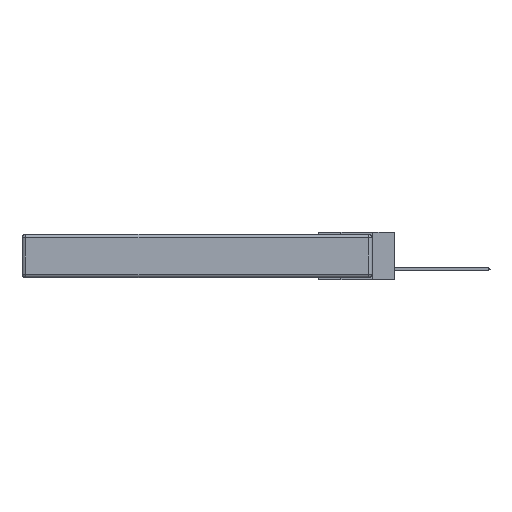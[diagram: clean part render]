
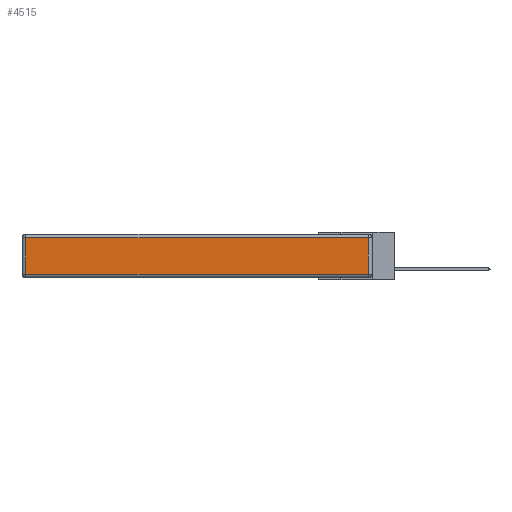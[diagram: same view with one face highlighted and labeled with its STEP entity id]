
A CAD part, left-side view. The second image highlights one B-rep face of the part: STEP entity #4515.
In plain terms, the highlighted planar face has unit normal (-1, 0, 0).
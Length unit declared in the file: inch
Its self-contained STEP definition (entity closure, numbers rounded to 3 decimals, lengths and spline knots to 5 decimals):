
#292 = ORIENTED_EDGE ( 'NONE', *, *, #18853, .T. ) ;
#667 = AXIS2_PLACEMENT_3D ( 'NONE', #30467, #11760, #16222 ) ;
#1671 = VERTEX_POINT ( 'NONE', #16600 ) ;
#2238 = DIRECTION ( 'NONE',  ( 0., -1., 0. ) ) ;
#3206 = VECTOR ( 'NONE', #18641, 39.37008 ) ;
#3739 = VERTEX_POINT ( 'NONE', #28798 ) ;
#4317 = VECTOR ( 'NONE', #6408, 39.37008 ) ;
#4515 = ADVANCED_FACE ( 'NONE', ( #8512 ), #11036, .T. ) ;
#5431 = EDGE_CURVE ( 'NONE', #5655, #1671, #20298, .T. ) ;
#5655 = VERTEX_POINT ( 'NONE', #28950 ) ;
#6261 = LINE ( 'NONE', #23536, #3206 ) ;
#6408 = DIRECTION ( 'NONE',  ( 0., 0., -1. ) ) ;
#6502 = ORIENTED_EDGE ( 'NONE', *, *, #24177, .T. ) ;
#6917 = CARTESIAN_POINT ( 'NONE',  ( 0., 0., -0.313 ) ) ;
#8512 = FACE_OUTER_BOUND ( 'NONE', #24902, .T. ) ;
#8844 = LINE ( 'NONE', #28328, #4317 ) ;
#9008 = CARTESIAN_POINT ( 'NONE',  ( 0., 2.72, -0.03 ) ) ;
#10210 = ORIENTED_EDGE ( 'NONE', *, *, #17461, .T. ) ;
#11036 = PLANE ( 'NONE',  #667 ) ;
#11760 = DIRECTION ( 'NONE',  ( -1., 0., 0. ) ) ;
#12027 = ORIENTED_EDGE ( 'NONE', *, *, #5431, .T. ) ;
#13085 = VECTOR ( 'NONE', #23020, 39.37008 ) ;
#14072 = VERTEX_POINT ( 'NONE', #9008 ) ;
#15008 = VECTOR ( 'NONE', #2238, 39.37008 ) ;
#16222 = DIRECTION ( 'NONE',  ( 0., 0., 1. ) ) ;
#16600 = CARTESIAN_POINT ( 'NONE',  ( 0., 0.03, -0.03 ) ) ;
#17461 = EDGE_CURVE ( 'NONE', #1671, #14072, #6261, .T. ) ;
#18641 = DIRECTION ( 'NONE',  ( 0., 1., 0. ) ) ;
#18853 = EDGE_CURVE ( 'NONE', #14072, #3739, #8844, .T. ) ;
#20298 = LINE ( 'NONE', #20932, #13085 ) ;
#20932 = CARTESIAN_POINT ( 'NONE',  ( 0., 0.03, -0.343 ) ) ;
#23020 = DIRECTION ( 'NONE',  ( 0., 0., 1. ) ) ;
#23536 = CARTESIAN_POINT ( 'NONE',  ( 0., 2.75, -0.03 ) ) ;
#24177 = EDGE_CURVE ( 'NONE', #3739, #5655, #27555, .T. ) ;
#24902 = EDGE_LOOP ( 'NONE', ( #6502, #12027, #10210, #292 ) ) ;
#27555 = LINE ( 'NONE', #6917, #15008 ) ;
#28328 = CARTESIAN_POINT ( 'NONE',  ( 0., 2.72, -0.343 ) ) ;
#28798 = CARTESIAN_POINT ( 'NONE',  ( 0., 2.72, -0.313 ) ) ;
#28950 = CARTESIAN_POINT ( 'NONE',  ( 0., 0.03, -0.313 ) ) ;
#30467 = CARTESIAN_POINT ( 'NONE',  ( 0., 0., -0.343 ) ) ;
